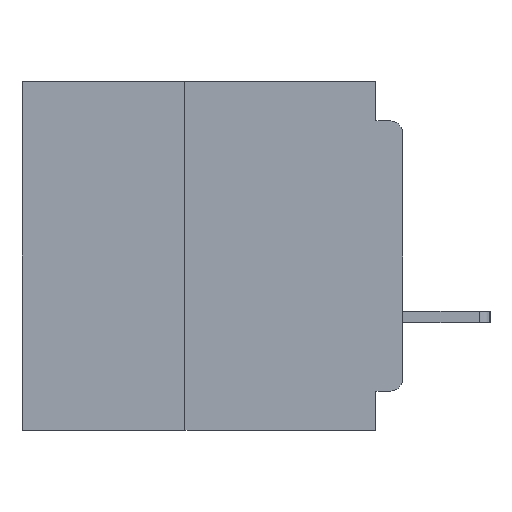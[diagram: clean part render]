
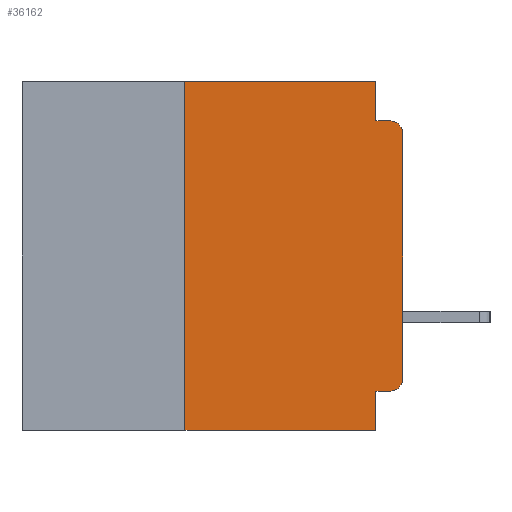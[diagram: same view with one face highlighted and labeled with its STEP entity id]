
A CAD part, left-side view. The second image highlights one B-rep face of the part: STEP entity #36162.
In plain terms, the highlighted planar face has unit normal (-1, 0, 0).
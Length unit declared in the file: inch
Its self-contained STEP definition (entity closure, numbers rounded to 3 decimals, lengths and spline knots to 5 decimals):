
#1859 = CARTESIAN_POINT ( 'NONE',  ( 0., 0.015, -0.045 ) ) ;
#3031 = VECTOR ( 'NONE', #13761, 39.37008 ) ;
#3934 = ORIENTED_EDGE ( 'NONE', *, *, #7016, .F. ) ;
#4013 = VECTOR ( 'NONE', #56837, 39.37008 ) ;
#4989 = DIRECTION ( 'NONE',  ( 0., 0., -1. ) ) ;
#5754 = DIRECTION ( 'NONE',  ( 0., -1., 0. ) ) ;
#6202 = LINE ( 'NONE', #26651, #47290 ) ;
#7016 = EDGE_CURVE ( 'NONE', #20819, #17946, #63385, .T. ) ;
#7259 = ORIENTED_EDGE ( 'NONE', *, *, #42587, .F. ) ;
#8037 = DIRECTION ( 'NONE',  ( 0., 0., 1. ) ) ;
#8363 = VECTOR ( 'NONE', #8037, 39.37008 ) ;
#8837 = CARTESIAN_POINT ( 'NONE',  ( 0., 0., 0. ) ) ;
#10117 = LINE ( 'NONE', #44726, #36978 ) ;
#10496 = EDGE_CURVE ( 'NONE', #18963, #45668, #39656, .T. ) ;
#10915 = AXIS2_PLACEMENT_3D ( 'NONE', #47599, #37082, #4989 ) ;
#13009 = VECTOR ( 'NONE', #16864, 39.37008 ) ;
#13347 = EDGE_LOOP ( 'NONE', ( #55572, #13836, #7259, #62179, #3934, #66746, #34904, #28107, #18473, #59453 ) ) ;
#13761 = DIRECTION ( 'NONE',  ( 0., -1., 0. ) ) ;
#13836 = ORIENTED_EDGE ( 'NONE', *, *, #63679, .T. ) ;
#14074 = AXIS2_PLACEMENT_3D ( 'NONE', #49375, #17332, #54765 ) ;
#16491 = FACE_OUTER_BOUND ( 'NONE', #13347, .T. ) ;
#16864 = DIRECTION ( 'NONE',  ( 0., 0., -1. ) ) ;
#17332 = DIRECTION ( 'NONE',  ( -1., 0., 0. ) ) ;
#17385 = VERTEX_POINT ( 'NONE', #63032 ) ;
#17946 = VERTEX_POINT ( 'NONE', #57072 ) ;
#18473 = ORIENTED_EDGE ( 'NONE', *, *, #10496, .F. ) ;
#18635 = EDGE_CURVE ( 'NONE', #17946, #63092, #27246, .T. ) ;
#18963 = VERTEX_POINT ( 'NONE', #41970 ) ;
#20819 = VERTEX_POINT ( 'NONE', #68389 ) ;
#21221 = DIRECTION ( 'NONE',  ( 0., 0., -1. ) ) ;
#21893 = EDGE_CURVE ( 'NONE', #18963, #58911, #39453, .T. ) ;
#22187 = DIRECTION ( 'NONE',  ( -1., 0., 0. ) ) ;
#24313 = LINE ( 'NONE', #45543, #8363 ) ;
#25343 = CARTESIAN_POINT ( 'NONE',  ( 0., 0.25, -0.4 ) ) ;
#25419 = VECTOR ( 'NONE', #47644, 39.37008 ) ;
#25554 = AXIS2_PLACEMENT_3D ( 'NONE', #54254, #22187, #59661 ) ;
#26124 = CARTESIAN_POINT ( 'NONE',  ( 0., 0., -0.355 ) ) ;
#26651 = CARTESIAN_POINT ( 'NONE',  ( 0., 0.031, -0.4 ) ) ;
#26843 = CARTESIAN_POINT ( 'NONE',  ( 0., 0.437, -0.4 ) ) ;
#27246 = LINE ( 'NONE', #59730, #13009 ) ;
#28107 = ORIENTED_EDGE ( 'NONE', *, *, #32209, .F. ) ;
#32209 = EDGE_CURVE ( 'NONE', #45668, #63909, #6202, .T. ) ;
#32475 = LINE ( 'NONE', #8837, #4013 ) ;
#34904 = ORIENTED_EDGE ( 'NONE', *, *, #55778, .T. ) ;
#35118 = CARTESIAN_POINT ( 'NONE',  ( 0., 0.437, 0. ) ) ;
#35915 = VECTOR ( 'NONE', #5754, 39.37008 ) ;
#36162 = ADVANCED_FACE ( 'NONE', ( #16491 ), #69119, .F. ) ;
#36978 = VECTOR ( 'NONE', #50054, 39.37008 ) ;
#37082 = DIRECTION ( 'NONE',  ( 1., 0., 0. ) ) ;
#39453 = CIRCLE ( 'NONE', #14074, 0.015 ) ;
#39656 = LINE ( 'NONE', #26124, #25419 ) ;
#41970 = CARTESIAN_POINT ( 'NONE',  ( 0., 0.015, -0.355 ) ) ;
#42587 = EDGE_CURVE ( 'NONE', #63092, #68404, #10117, .T. ) ;
#44133 = VERTEX_POINT ( 'NONE', #25343 ) ;
#44726 = CARTESIAN_POINT ( 'NONE',  ( 0., 0., -0.045 ) ) ;
#45543 = CARTESIAN_POINT ( 'NONE',  ( 0., 0.25, -0.4 ) ) ;
#45668 = VERTEX_POINT ( 'NONE', #53739 ) ;
#47290 = VECTOR ( 'NONE', #21221, 39.37008 ) ;
#47599 = CARTESIAN_POINT ( 'NONE',  ( 0., 0.437, 0. ) ) ;
#47644 = DIRECTION ( 'NONE',  ( 0., 1., 0. ) ) ;
#48257 = CARTESIAN_POINT ( 'NONE',  ( 0., 0.031, -0.045 ) ) ;
#48275 = CIRCLE ( 'NONE', #25554, 0.015 ) ;
#49375 = CARTESIAN_POINT ( 'NONE',  ( 0., 0.015, -0.34 ) ) ;
#50054 = DIRECTION ( 'NONE',  ( 0., -1., 0. ) ) ;
#51782 = LINE ( 'NONE', #26843, #35915 ) ;
#52265 = EDGE_CURVE ( 'NONE', #58911, #17385, #32475, .T. ) ;
#53739 = CARTESIAN_POINT ( 'NONE',  ( 0., 0.031, -0.355 ) ) ;
#54254 = CARTESIAN_POINT ( 'NONE',  ( 0., 0.015, -0.06 ) ) ;
#54765 = DIRECTION ( 'NONE',  ( 0., 0., -1. ) ) ;
#55572 = ORIENTED_EDGE ( 'NONE', *, *, #52265, .T. ) ;
#55778 = EDGE_CURVE ( 'NONE', #44133, #63909, #51782, .T. ) ;
#56837 = DIRECTION ( 'NONE',  ( 0., 0., 1. ) ) ;
#57072 = CARTESIAN_POINT ( 'NONE',  ( 0., 0.031, 0. ) ) ;
#58911 = VERTEX_POINT ( 'NONE', #68735 ) ;
#59453 = ORIENTED_EDGE ( 'NONE', *, *, #21893, .T. ) ;
#59661 = DIRECTION ( 'NONE',  ( 0., 0., -1. ) ) ;
#59730 = CARTESIAN_POINT ( 'NONE',  ( 0., 0.031, 0. ) ) ;
#60993 = EDGE_CURVE ( 'NONE', #44133, #20819, #24313, .T. ) ;
#62179 = ORIENTED_EDGE ( 'NONE', *, *, #18635, .F. ) ;
#63032 = CARTESIAN_POINT ( 'NONE',  ( 0., 0., -0.06 ) ) ;
#63092 = VERTEX_POINT ( 'NONE', #48257 ) ;
#63385 = LINE ( 'NONE', #35118, #3031 ) ;
#63679 = EDGE_CURVE ( 'NONE', #17385, #68404, #48275, .T. ) ;
#63909 = VERTEX_POINT ( 'NONE', #68019 ) ;
#66746 = ORIENTED_EDGE ( 'NONE', *, *, #60993, .F. ) ;
#68019 = CARTESIAN_POINT ( 'NONE',  ( 0., 0.031, -0.4 ) ) ;
#68389 = CARTESIAN_POINT ( 'NONE',  ( 0., 0.25, 0. ) ) ;
#68404 = VERTEX_POINT ( 'NONE', #1859 ) ;
#68735 = CARTESIAN_POINT ( 'NONE',  ( 0., 0., -0.34 ) ) ;
#69119 = PLANE ( 'NONE',  #10915 ) ;
